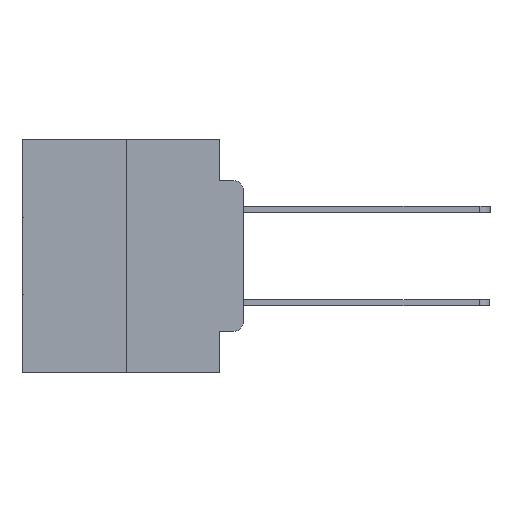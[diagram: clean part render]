
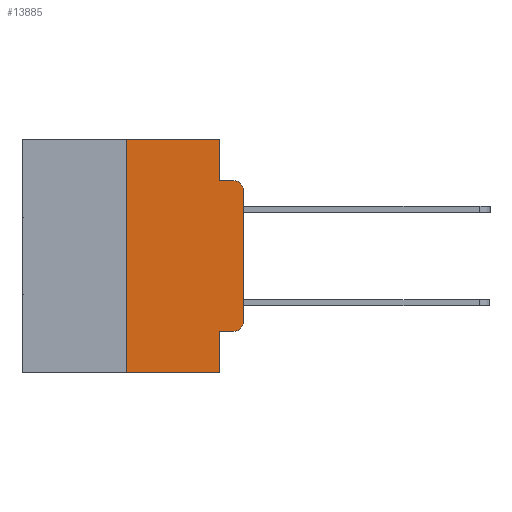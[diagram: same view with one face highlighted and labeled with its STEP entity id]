
A CAD part, left-side view. The second image highlights one B-rep face of the part: STEP entity #13885.
In plain terms, the highlighted planar face has unit normal (-1, 0, 0).
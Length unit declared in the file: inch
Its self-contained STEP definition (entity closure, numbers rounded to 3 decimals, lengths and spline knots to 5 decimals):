
#130 = VERTEX_POINT ( 'NONE', #7494 ) ;
#365 = LINE ( 'NONE', #14630, #24126 ) ;
#779 = LINE ( 'NONE', #13143, #6260 ) ;
#865 = DIRECTION ( 'NONE',  ( 0., 0., -1. ) ) ;
#884 = DIRECTION ( 'NONE',  ( -1., 0., 0. ) ) ;
#1045 = VECTOR ( 'NONE', #12272, 39.37008 ) ;
#1776 = LINE ( 'NONE', #9955, #1045 ) ;
#1821 = CARTESIAN_POINT ( 'NONE',  ( 0., 0.02, -0.1085 ) ) ;
#1834 = CARTESIAN_POINT ( 'NONE',  ( 0., 0.25, 0. ) ) ;
#2019 = CARTESIAN_POINT ( 'NONE',  ( 0., 0.25, 0. ) ) ;
#2350 = EDGE_CURVE ( 'NONE', #4766, #26121, #365, .T. ) ;
#2784 = CARTESIAN_POINT ( 'NONE',  ( 0., 0.473, 0. ) ) ;
#3081 = CARTESIAN_POINT ( 'NONE',  ( 0., 0., 0. ) ) ;
#4079 = ORIENTED_EDGE ( 'NONE', *, *, #11449, .T. ) ;
#4182 = DIRECTION ( 'NONE',  ( 0., 0., -1. ) ) ;
#4296 = DIRECTION ( 'NONE',  ( 0., 0., 1. ) ) ;
#4681 = EDGE_CURVE ( 'NONE', #18825, #22417, #15498, .T. ) ;
#4766 = VERTEX_POINT ( 'NONE', #21931 ) ;
#5323 = VERTEX_POINT ( 'NONE', #5640 ) ;
#5474 = VECTOR ( 'NONE', #26039, 39.37008 ) ;
#5507 = ORIENTED_EDGE ( 'NONE', *, *, #20114, .F. ) ;
#5640 = CARTESIAN_POINT ( 'NONE',  ( 0., 0.051, -0.4115 ) ) ;
#6237 = EDGE_CURVE ( 'NONE', #22417, #14127, #8593, .T. ) ;
#6260 = VECTOR ( 'NONE', #20017, 39.37008 ) ;
#7470 = PLANE ( 'NONE',  #19965 ) ;
#7494 = CARTESIAN_POINT ( 'NONE',  ( 0., 0., -0.1085 ) ) ;
#7850 = VECTOR ( 'NONE', #4296, 39.37008 ) ;
#8376 = CARTESIAN_POINT ( 'NONE',  ( 0., 0.02, -0.0885 ) ) ;
#8579 = VERTEX_POINT ( 'NONE', #27954 ) ;
#8593 = LINE ( 'NONE', #21981, #13251 ) ;
#8796 = ORIENTED_EDGE ( 'NONE', *, *, #13014, .T. ) ;
#9955 = CARTESIAN_POINT ( 'NONE',  ( 0., 0.051, 0. ) ) ;
#11049 = CARTESIAN_POINT ( 'NONE',  ( 0., 0.051, -0.0885 ) ) ;
#11449 = EDGE_CURVE ( 'NONE', #14222, #8579, #18554, .T. ) ;
#12272 = DIRECTION ( 'NONE',  ( 0., 0., -1. ) ) ;
#12312 = DIRECTION ( 'NONE',  ( 0., -1., 0. ) ) ;
#12438 = EDGE_CURVE ( 'NONE', #130, #14127, #28384, .T. ) ;
#12606 = VECTOR ( 'NONE', #865, 39.37008 ) ;
#13014 = EDGE_CURVE ( 'NONE', #5323, #14222, #779, .T. ) ;
#13143 = CARTESIAN_POINT ( 'NONE',  ( 0., 0.051, -0.4115 ) ) ;
#13251 = VECTOR ( 'NONE', #17425, 39.37008 ) ;
#13885 = ADVANCED_FACE ( 'NONE', ( #26579 ), #7470, .F. ) ;
#13978 = EDGE_CURVE ( 'NONE', #8579, #130, #19154, .T. ) ;
#14127 = VERTEX_POINT ( 'NONE', #8376 ) ;
#14222 = VERTEX_POINT ( 'NONE', #29240 ) ;
#14435 = DIRECTION ( 'NONE',  ( 0., 0., -1. ) ) ;
#14562 = EDGE_CURVE ( 'NONE', #5323, #26121, #1776, .T. ) ;
#14630 = CARTESIAN_POINT ( 'NONE',  ( 0., 0.473, -0.5 ) ) ;
#14680 = CARTESIAN_POINT ( 'NONE',  ( 0., 0.051, 0. ) ) ;
#14801 = CARTESIAN_POINT ( 'NONE',  ( 0., 0.02, -0.3915 ) ) ;
#15498 = LINE ( 'NONE', #26170, #12606 ) ;
#15984 = ORIENTED_EDGE ( 'NONE', *, *, #2350, .T. ) ;
#16022 = ORIENTED_EDGE ( 'NONE', *, *, #4681, .F. ) ;
#16339 = LINE ( 'NONE', #19481, #27649 ) ;
#17094 = DIRECTION ( 'NONE',  ( 0., 0., -1. ) ) ;
#17372 = EDGE_LOOP ( 'NONE', ( #28370, #29405, #29096, #16022, #5507, #24487, #15984, #28744, #8796, #4079 ) ) ;
#17425 = DIRECTION ( 'NONE',  ( 0., -1., 0. ) ) ;
#17996 = DIRECTION ( 'NONE',  ( -1., 0., 0. ) ) ;
#18554 = CIRCLE ( 'NONE', #24489, 0.02 ) ;
#18825 = VERTEX_POINT ( 'NONE', #14680 ) ;
#19154 = LINE ( 'NONE', #3081, #5474 ) ;
#19383 = DIRECTION ( 'NONE',  ( 0., -1., 0. ) ) ;
#19481 = CARTESIAN_POINT ( 'NONE',  ( 0., 0.473, 0. ) ) ;
#19965 = AXIS2_PLACEMENT_3D ( 'NONE', #2784, #27983, #14435 ) ;
#20017 = DIRECTION ( 'NONE',  ( 0., -1., 0. ) ) ;
#20114 = EDGE_CURVE ( 'NONE', #20384, #18825, #16339, .T. ) ;
#20384 = VERTEX_POINT ( 'NONE', #2019 ) ;
#21931 = CARTESIAN_POINT ( 'NONE',  ( 0., 0.25, -0.5 ) ) ;
#21981 = CARTESIAN_POINT ( 'NONE',  ( 0., 0.051, -0.0885 ) ) ;
#22417 = VERTEX_POINT ( 'NONE', #11049 ) ;
#23691 = EDGE_CURVE ( 'NONE', #4766, #20384, #26054, .T. ) ;
#24126 = VECTOR ( 'NONE', #12312, 39.37008 ) ;
#24312 = AXIS2_PLACEMENT_3D ( 'NONE', #1821, #17996, #4182 ) ;
#24487 = ORIENTED_EDGE ( 'NONE', *, *, #23691, .F. ) ;
#24489 = AXIS2_PLACEMENT_3D ( 'NONE', #14801, #884, #17094 ) ;
#26039 = DIRECTION ( 'NONE',  ( 0., 0., 1. ) ) ;
#26054 = LINE ( 'NONE', #1834, #7850 ) ;
#26121 = VERTEX_POINT ( 'NONE', #26767 ) ;
#26170 = CARTESIAN_POINT ( 'NONE',  ( 0., 0.051, 0. ) ) ;
#26579 = FACE_OUTER_BOUND ( 'NONE', #17372, .T. ) ;
#26767 = CARTESIAN_POINT ( 'NONE',  ( 0., 0.051, -0.5 ) ) ;
#27649 = VECTOR ( 'NONE', #19383, 39.37008 ) ;
#27954 = CARTESIAN_POINT ( 'NONE',  ( 0., 0., -0.3915 ) ) ;
#27983 = DIRECTION ( 'NONE',  ( 1., 0., 0. ) ) ;
#28370 = ORIENTED_EDGE ( 'NONE', *, *, #13978, .T. ) ;
#28384 = CIRCLE ( 'NONE', #24312, 0.02 ) ;
#28744 = ORIENTED_EDGE ( 'NONE', *, *, #14562, .F. ) ;
#29096 = ORIENTED_EDGE ( 'NONE', *, *, #6237, .F. ) ;
#29240 = CARTESIAN_POINT ( 'NONE',  ( 0., 0.02, -0.4115 ) ) ;
#29405 = ORIENTED_EDGE ( 'NONE', *, *, #12438, .T. ) ;
